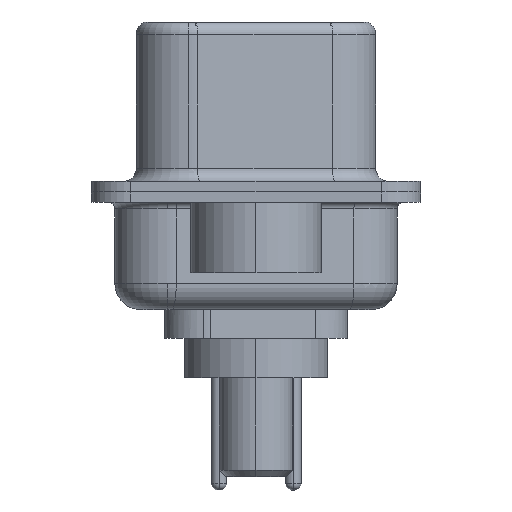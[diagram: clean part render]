
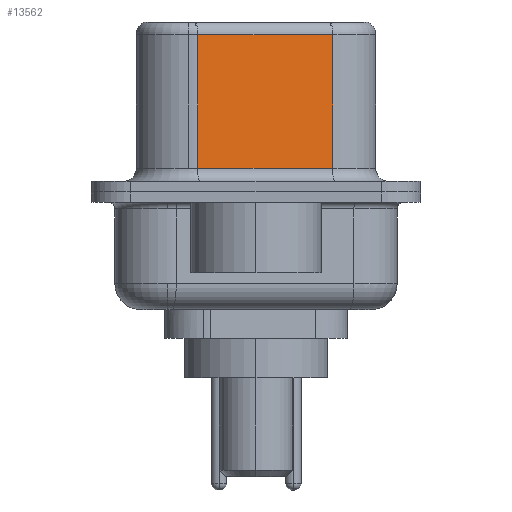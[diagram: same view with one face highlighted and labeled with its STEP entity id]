
A CAD part, left-side view. The second image highlights one B-rep face of the part: STEP entity #13562.
In plain terms, the highlighted planar face has unit normal (-0.985, -0.174, 0).
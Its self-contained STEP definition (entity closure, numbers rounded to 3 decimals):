
#143 = LINE ( 'NONE', #16885, #17506 ) ;
#712 = CARTESIAN_POINT ( 'NONE',  ( 4.58, -2.927, 6.52 ) ) ;
#775 = ORIENTED_EDGE ( 'NONE', *, *, #16634, .F. ) ;
#782 = ORIENTED_EDGE ( 'NONE', *, *, #11690, .T. ) ;
#1417 = CARTESIAN_POINT ( 'NONE',  ( 3.67, 2.233, 6.52 ) ) ;
#2592 = VECTOR ( 'NONE', #10353, 1000. ) ;
#4061 = ORIENTED_EDGE ( 'NONE', *, *, #17066, .T. ) ;
#4321 = CARTESIAN_POINT ( 'NONE',  ( 4.58, -2.927, 0.9 ) ) ;
#5235 = CARTESIAN_POINT ( 'NONE',  ( 4.58, -2.927, 6.02 ) ) ;
#5312 = LINE ( 'NONE', #14483, #17688 ) ;
#6830 = DIRECTION ( 'NONE',  ( 0.174, -0.985, 0. ) ) ;
#7492 = PLANE ( 'NONE',  #11903 ) ;
#9177 = DIRECTION ( 'NONE',  ( -0.174, 0.985, 0. ) ) ;
#9791 = VECTOR ( 'NONE', #13184, 1000. ) ;
#10071 = EDGE_LOOP ( 'NONE', ( #775, #782, #4061, #17167 ) ) ;
#10353 = DIRECTION ( 'NONE',  ( -0.174, 0.985, 0. ) ) ;
#10468 = VERTEX_POINT ( 'NONE', #15397 ) ;
#11553 = LINE ( 'NONE', #5235, #2592 ) ;
#11690 = EDGE_CURVE ( 'NONE', #20922, #19189, #11553, .T. ) ;
#11903 = AXIS2_PLACEMENT_3D ( 'NONE', #712, #19282, #9177 ) ;
#13184 = DIRECTION ( 'NONE',  ( 0., 0., -1. ) ) ;
#13272 = EDGE_CURVE ( 'NONE', #10468, #13628, #143, .T. ) ;
#13562 = ADVANCED_FACE ( 'NONE', ( #17768 ), #7492, .F. ) ;
#13628 = VERTEX_POINT ( 'NONE', #4321 ) ;
#14245 = LINE ( 'NONE', #1417, #9791 ) ;
#14483 = CARTESIAN_POINT ( 'NONE',  ( 4.58, -2.927, 6.52 ) ) ;
#15397 = CARTESIAN_POINT ( 'NONE',  ( 3.67, 2.233, 0.9 ) ) ;
#16163 = DIRECTION ( 'NONE',  ( 0., 0., -1. ) ) ;
#16634 = EDGE_CURVE ( 'NONE', #20922, #13628, #5312, .T. ) ;
#16885 = CARTESIAN_POINT ( 'NONE',  ( 4.58, -2.927, 0.9 ) ) ;
#17066 = EDGE_CURVE ( 'NONE', #19189, #10468, #14245, .T. ) ;
#17094 = CARTESIAN_POINT ( 'NONE',  ( 4.58, -2.927, 6.02 ) ) ;
#17167 = ORIENTED_EDGE ( 'NONE', *, *, #13272, .T. ) ;
#17506 = VECTOR ( 'NONE', #6830, 1000. ) ;
#17688 = VECTOR ( 'NONE', #16163, 1000. ) ;
#17768 = FACE_OUTER_BOUND ( 'NONE', #10071, .T. ) ;
#18749 = CARTESIAN_POINT ( 'NONE',  ( 3.67, 2.233, 6.02 ) ) ;
#19189 = VERTEX_POINT ( 'NONE', #18749 ) ;
#19282 = DIRECTION ( 'NONE',  ( 0.985, 0.174, 0. ) ) ;
#20922 = VERTEX_POINT ( 'NONE', #17094 ) ;
